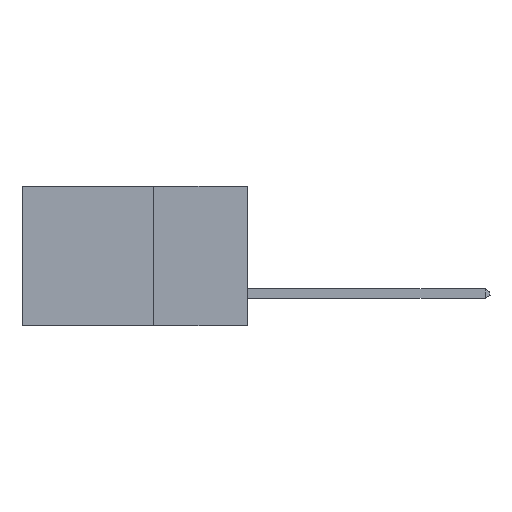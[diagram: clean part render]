
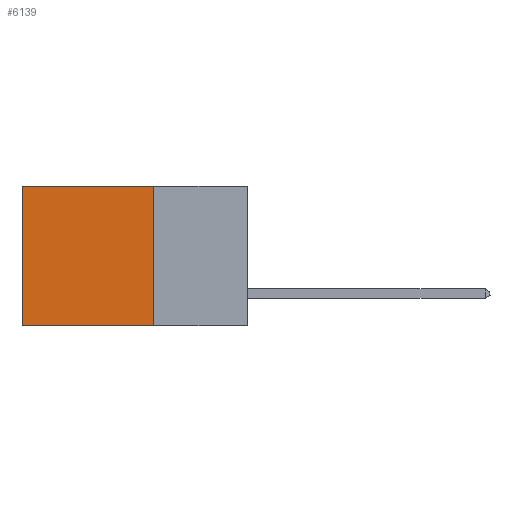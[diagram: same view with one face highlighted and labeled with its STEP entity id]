
A CAD part, left-side view. The second image highlights one B-rep face of the part: STEP entity #6139.
In plain terms, the highlighted planar face has unit normal (-1, 0, 0).
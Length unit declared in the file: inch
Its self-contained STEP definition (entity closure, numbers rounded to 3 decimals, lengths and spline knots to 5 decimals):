
#1879 = CARTESIAN_POINT ( 'NONE',  ( 0.298, 0.25, 0. ) ) ;
#2667 = LINE ( 'NONE', #7801, #19055 ) ;
#2812 = ORIENTED_EDGE ( 'NONE', *, *, #13628, .F. ) ;
#5342 = CARTESIAN_POINT ( 'NONE',  ( 0.298, 0.25, -0.37 ) ) ;
#5344 = DIRECTION ( 'NONE',  ( 0., 0., -1. ) ) ;
#5393 = DIRECTION ( 'NONE',  ( 0., 0., -1. ) ) ;
#6139 = ADVANCED_FACE ( 'NONE', ( #21341 ), #10305, .F. ) ;
#6942 = ORIENTED_EDGE ( 'NONE', *, *, #18942, .T. ) ;
#7383 = LINE ( 'NONE', #1879, #21334 ) ;
#7801 = CARTESIAN_POINT ( 'NONE',  ( 0.298, 0.25, -0.37 ) ) ;
#8371 = AXIS2_PLACEMENT_3D ( 'NONE', #17475, #12165, #5344 ) ;
#8865 = CARTESIAN_POINT ( 'NONE',  ( 0.298, 0.25, 0. ) ) ;
#9871 = CARTESIAN_POINT ( 'NONE',  ( 0.298, 0.6, 0. ) ) ;
#10070 = ORIENTED_EDGE ( 'NONE', *, *, #16847, .F. ) ;
#10305 = PLANE ( 'NONE',  #8371 ) ;
#10325 = ORIENTED_EDGE ( 'NONE', *, *, #13558, .T. ) ;
#11248 = DIRECTION ( 'NONE',  ( 0., 1., 0. ) ) ;
#11507 = VERTEX_POINT ( 'NONE', #14351 ) ;
#11549 = VECTOR ( 'NONE', #5393, 39.37008 ) ;
#12165 = DIRECTION ( 'NONE',  ( 1., 0., 0. ) ) ;
#12769 = EDGE_LOOP ( 'NONE', ( #10325, #10070, #2812, #6942 ) ) ;
#13005 = VERTEX_POINT ( 'NONE', #8865 ) ;
#13558 = EDGE_CURVE ( 'NONE', #14876, #11507, #16176, .T. ) ;
#13628 = EDGE_CURVE ( 'NONE', #13005, #21239, #19496, .T. ) ;
#14126 = DIRECTION ( 'NONE',  ( 0., 1., 0. ) ) ;
#14132 = CARTESIAN_POINT ( 'NONE',  ( 0.298, 0.6, 0. ) ) ;
#14351 = CARTESIAN_POINT ( 'NONE',  ( 0.298, 0.6, -0.37 ) ) ;
#14876 = VERTEX_POINT ( 'NONE', #9871 ) ;
#16176 = LINE ( 'NONE', #14132, #11549 ) ;
#16847 = EDGE_CURVE ( 'NONE', #21239, #11507, #2667, .T. ) ;
#17475 = CARTESIAN_POINT ( 'NONE',  ( 0.298, 0.25, 0. ) ) ;
#18942 = EDGE_CURVE ( 'NONE', #13005, #14876, #7383, .T. ) ;
#19055 = VECTOR ( 'NONE', #11248, 39.37008 ) ;
#19496 = LINE ( 'NONE', #21028, #21928 ) ;
#19603 = DIRECTION ( 'NONE',  ( 0., 0., -1. ) ) ;
#21028 = CARTESIAN_POINT ( 'NONE',  ( 0.298, 0.25, 0. ) ) ;
#21239 = VERTEX_POINT ( 'NONE', #5342 ) ;
#21334 = VECTOR ( 'NONE', #14126, 39.37008 ) ;
#21341 = FACE_OUTER_BOUND ( 'NONE', #12769, .T. ) ;
#21928 = VECTOR ( 'NONE', #19603, 39.37008 ) ;
